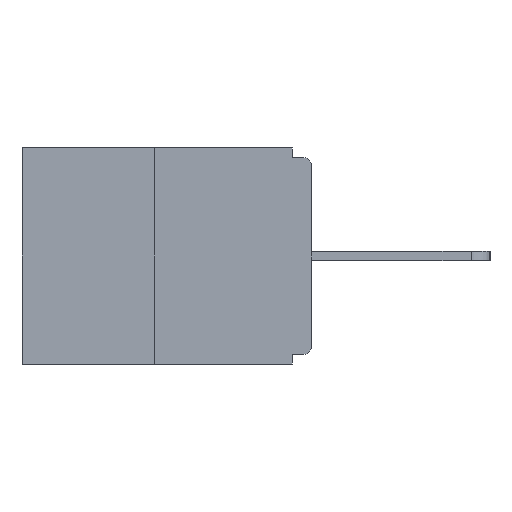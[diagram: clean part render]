
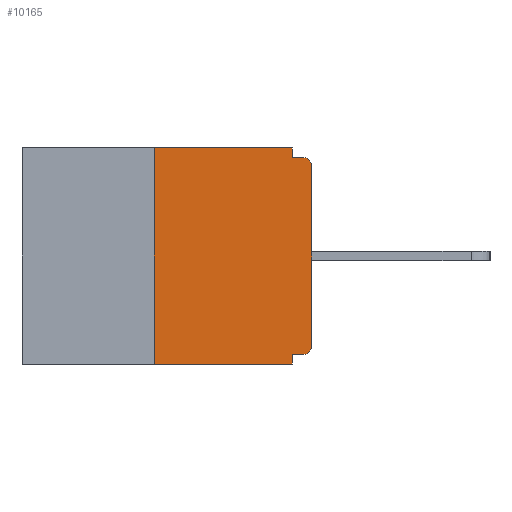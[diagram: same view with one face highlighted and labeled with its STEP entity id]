
A CAD part, left-side view. The second image highlights one B-rep face of the part: STEP entity #10165.
In plain terms, the highlighted planar face has unit normal (-1, 0, 0).
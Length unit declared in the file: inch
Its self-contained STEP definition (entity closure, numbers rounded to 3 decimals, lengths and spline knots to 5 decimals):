
#47 = CARTESIAN_POINT ( 'NONE',  ( 0., 0.25, 0. ) ) ;
#112 = VECTOR ( 'NONE', #5441, 39.37008 ) ;
#146 = ORIENTED_EDGE ( 'NONE', *, *, #9222, .F. ) ;
#382 = PLANE ( 'NONE',  #4182 ) ;
#474 = DIRECTION ( 'NONE',  ( 0., 0., -1. ) ) ;
#506 = LINE ( 'NONE', #4444, #12444 ) ;
#521 = DIRECTION ( 'NONE',  ( 1., 0., 0. ) ) ;
#527 = VECTOR ( 'NONE', #10873, 39.37008 ) ;
#745 = CARTESIAN_POINT ( 'NONE',  ( 0., 0., -0.015 ) ) ;
#967 = ORIENTED_EDGE ( 'NONE', *, *, #9852, .F. ) ;
#1014 = VERTEX_POINT ( 'NONE', #47 ) ;
#2123 = DIRECTION ( 'NONE',  ( 0., 0., -1. ) ) ;
#2229 = CARTESIAN_POINT ( 'NONE',  ( 0., 0.031, 0. ) ) ;
#2461 = VERTEX_POINT ( 'NONE', #2905 ) ;
#2515 = EDGE_CURVE ( 'NONE', #2461, #8228, #7931, .T. ) ;
#2689 = LINE ( 'NONE', #9713, #10051 ) ;
#2699 = CARTESIAN_POINT ( 'NONE',  ( 0., 0.015, -0.328 ) ) ;
#2715 = CARTESIAN_POINT ( 'NONE',  ( 0., 0., 0. ) ) ;
#2768 = LINE ( 'NONE', #745, #5464 ) ;
#2905 = CARTESIAN_POINT ( 'NONE',  ( 0., 0.031, -0.328 ) ) ;
#2916 = CARTESIAN_POINT ( 'NONE',  ( 0., 0.031, 0. ) ) ;
#3167 = LINE ( 'NONE', #10545, #112 ) ;
#3447 = CARTESIAN_POINT ( 'NONE',  ( 0., 0.25, -0.343 ) ) ;
#3543 = AXIS2_PLACEMENT_3D ( 'NONE', #9928, #10999, #474 ) ;
#3595 = ORIENTED_EDGE ( 'NONE', *, *, #10361, .F. ) ;
#3942 = DIRECTION ( 'NONE',  ( 0., -1., 0. ) ) ;
#4101 = CARTESIAN_POINT ( 'NONE',  ( 0., 0.031, -0.015 ) ) ;
#4182 = AXIS2_PLACEMENT_3D ( 'NONE', #10711, #521, #12531 ) ;
#4338 = VERTEX_POINT ( 'NONE', #5333 ) ;
#4351 = CARTESIAN_POINT ( 'NONE',  ( 0., 0.46, 0. ) ) ;
#4444 = CARTESIAN_POINT ( 'NONE',  ( 0., 0.46, -0.343 ) ) ;
#4556 = CIRCLE ( 'NONE', #10342, 0.015 ) ;
#4760 = EDGE_CURVE ( 'NONE', #4837, #8228, #506, .T. ) ;
#4837 = VERTEX_POINT ( 'NONE', #3447 ) ;
#4938 = DIRECTION ( 'NONE',  ( -1., 0., 0. ) ) ;
#5241 = CIRCLE ( 'NONE', #3543, 0.015 ) ;
#5275 = ORIENTED_EDGE ( 'NONE', *, *, #6740, .F. ) ;
#5333 = CARTESIAN_POINT ( 'NONE',  ( 0., 0., -0.313 ) ) ;
#5441 = DIRECTION ( 'NONE',  ( 0., 1., 0. ) ) ;
#5464 = VECTOR ( 'NONE', #3942, 39.37008 ) ;
#5685 = EDGE_CURVE ( 'NONE', #4837, #1014, #2689, .T. ) ;
#5977 = CARTESIAN_POINT ( 'NONE',  ( 0., 0.031, -0.343 ) ) ;
#6314 = LINE ( 'NONE', #4351, #12988 ) ;
#6614 = VERTEX_POINT ( 'NONE', #2916 ) ;
#6702 = VERTEX_POINT ( 'NONE', #7327 ) ;
#6740 = EDGE_CURVE ( 'NONE', #6614, #11686, #9263, .T. ) ;
#7327 = CARTESIAN_POINT ( 'NONE',  ( 0., 0.015, -0.015 ) ) ;
#7823 = DIRECTION ( 'NONE',  ( 0., -1., 0. ) ) ;
#7836 = EDGE_LOOP ( 'NONE', ( #3595, #11629, #10648, #11715, #146, #8062, #9643, #10374, #967, #5275 ) ) ;
#7931 = LINE ( 'NONE', #12015, #10090 ) ;
#8058 = CARTESIAN_POINT ( 'NONE',  ( 0., 0., -0.03 ) ) ;
#8062 = ORIENTED_EDGE ( 'NONE', *, *, #12414, .T. ) ;
#8228 = VERTEX_POINT ( 'NONE', #5977 ) ;
#8273 = EDGE_CURVE ( 'NONE', #4338, #12074, #9938, .T. ) ;
#8513 = FACE_OUTER_BOUND ( 'NONE', #7836, .T. ) ;
#8584 = VERTEX_POINT ( 'NONE', #2699 ) ;
#9222 = EDGE_CURVE ( 'NONE', #8584, #2461, #3167, .T. ) ;
#9263 = LINE ( 'NONE', #2229, #12006 ) ;
#9643 = ORIENTED_EDGE ( 'NONE', *, *, #8273, .T. ) ;
#9713 = CARTESIAN_POINT ( 'NONE',  ( 0., 0.25, 0. ) ) ;
#9852 = EDGE_CURVE ( 'NONE', #11686, #6702, #2768, .T. ) ;
#9928 = CARTESIAN_POINT ( 'NONE',  ( 0., 0.015, -0.03 ) ) ;
#9938 = LINE ( 'NONE', #2715, #527 ) ;
#10051 = VECTOR ( 'NONE', #12803, 39.37008 ) ;
#10090 = VECTOR ( 'NONE', #11465, 39.37008 ) ;
#10165 = ADVANCED_FACE ( 'NONE', ( #8513 ), #382, .F. ) ;
#10266 = DIRECTION ( 'NONE',  ( 0., 0., -1. ) ) ;
#10342 = AXIS2_PLACEMENT_3D ( 'NONE', #12185, #4938, #2123 ) ;
#10361 = EDGE_CURVE ( 'NONE', #1014, #6614, #6314, .T. ) ;
#10374 = ORIENTED_EDGE ( 'NONE', *, *, #10595, .T. ) ;
#10545 = CARTESIAN_POINT ( 'NONE',  ( 0., 0., -0.328 ) ) ;
#10595 = EDGE_CURVE ( 'NONE', #12074, #6702, #5241, .T. ) ;
#10648 = ORIENTED_EDGE ( 'NONE', *, *, #4760, .T. ) ;
#10711 = CARTESIAN_POINT ( 'NONE',  ( 0., 0.46, 0. ) ) ;
#10873 = DIRECTION ( 'NONE',  ( 0., 0., 1. ) ) ;
#10999 = DIRECTION ( 'NONE',  ( -1., 0., 0. ) ) ;
#11465 = DIRECTION ( 'NONE',  ( 0., 0., -1. ) ) ;
#11629 = ORIENTED_EDGE ( 'NONE', *, *, #5685, .F. ) ;
#11686 = VERTEX_POINT ( 'NONE', #4101 ) ;
#11715 = ORIENTED_EDGE ( 'NONE', *, *, #2515, .F. ) ;
#12006 = VECTOR ( 'NONE', #10266, 39.37008 ) ;
#12015 = CARTESIAN_POINT ( 'NONE',  ( 0., 0.031, -0.343 ) ) ;
#12074 = VERTEX_POINT ( 'NONE', #8058 ) ;
#12185 = CARTESIAN_POINT ( 'NONE',  ( 0., 0.015, -0.313 ) ) ;
#12414 = EDGE_CURVE ( 'NONE', #8584, #4338, #4556, .T. ) ;
#12444 = VECTOR ( 'NONE', #7823, 39.37008 ) ;
#12531 = DIRECTION ( 'NONE',  ( 0., 0., -1. ) ) ;
#12686 = DIRECTION ( 'NONE',  ( 0., -1., 0. ) ) ;
#12803 = DIRECTION ( 'NONE',  ( 0., 0., 1. ) ) ;
#12988 = VECTOR ( 'NONE', #12686, 39.37008 ) ;
